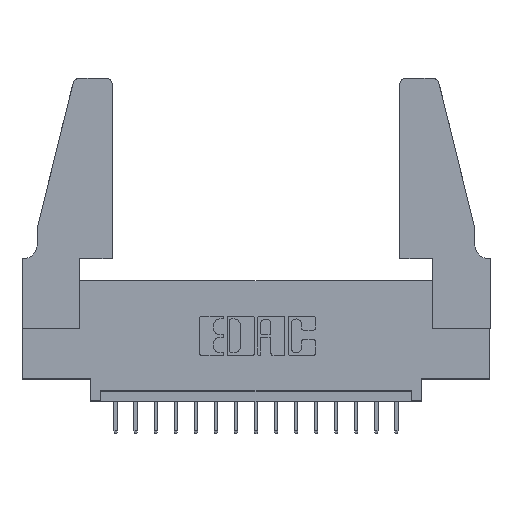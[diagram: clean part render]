
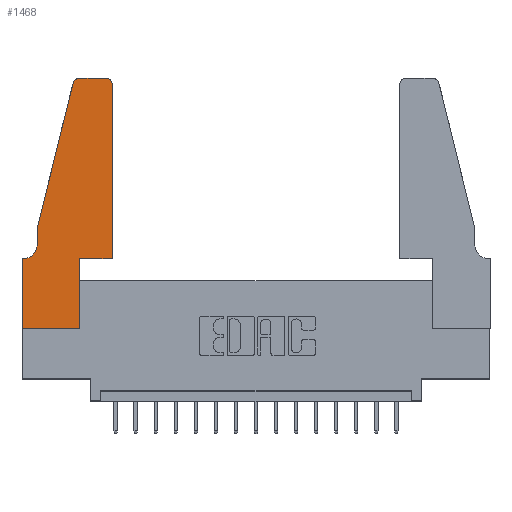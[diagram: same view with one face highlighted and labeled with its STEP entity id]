
A CAD part, top view. The second image highlights one B-rep face of the part: STEP entity #1468.
In plain terms, the highlighted planar face has unit normal (0, 0, 1).
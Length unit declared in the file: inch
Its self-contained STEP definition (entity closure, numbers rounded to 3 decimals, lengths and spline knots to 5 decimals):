
#71 = DIRECTION ( 'NONE',  ( -0.239, -0.971, 0. ) ) ;
#103 = DIRECTION ( 'NONE',  ( 0., 0., 1. ) ) ;
#128 = ORIENTED_EDGE ( 'NONE', *, *, #11020, .T. ) ;
#147 = VERTEX_POINT ( 'NONE', #17184 ) ;
#299 = ORIENTED_EDGE ( 'NONE', *, *, #2047, .T. ) ;
#352 = VERTEX_POINT ( 'NONE', #2187 ) ;
#450 = DIRECTION ( 'NONE',  ( 1., 0., 0. ) ) ;
#629 = EDGE_CURVE ( 'NONE', #147, #1503, #12764, .T. ) ;
#857 = DIRECTION ( 'NONE',  ( 0., 0., 1. ) ) ;
#936 = DIRECTION ( 'NONE',  ( 1., 0., 0. ) ) ;
#990 = VECTOR ( 'NONE', #10093, 39.37008 ) ;
#1235 = DIRECTION ( 'NONE',  ( 0., -1., 0. ) ) ;
#1468 = ADVANCED_FACE ( 'NONE', ( #2275 ), #4804, .T. ) ;
#1503 = VERTEX_POINT ( 'NONE', #3498 ) ;
#1647 = ORIENTED_EDGE ( 'NONE', *, *, #12809, .T. ) ;
#1787 = CARTESIAN_POINT ( 'NONE',  ( 0.0055, 0.42, 0.37 ) ) ;
#2047 = EDGE_CURVE ( 'NONE', #6552, #7746, #2246, .T. ) ;
#2187 = CARTESIAN_POINT ( 'NONE',  ( 0.0755, 0.42, 0.37 ) ) ;
#2246 = LINE ( 'NONE', #8787, #990 ) ;
#2275 = FACE_OUTER_BOUND ( 'NONE', #10332, .T. ) ;
#2312 = CARTESIAN_POINT ( 'NONE',  ( 0.2865, 0.35, 0.37 ) ) ;
#2389 = ORIENTED_EDGE ( 'NONE', *, *, #8992, .T. ) ;
#2421 = EDGE_CURVE ( 'NONE', #13683, #147, #16655, .T. ) ;
#2597 = LINE ( 'NONE', #13970, #16398 ) ;
#2648 = CARTESIAN_POINT ( 'NONE',  ( 0.2865, 0., 0.37 ) ) ;
#3378 = CARTESIAN_POINT ( 'NONE',  ( 0.4505, 0.35, 0.37 ) ) ;
#3498 = CARTESIAN_POINT ( 'NONE',  ( 0.0755, 0.5, 0.37 ) ) ;
#3772 = EDGE_CURVE ( 'NONE', #4771, #9372, #8177, .T. ) ;
#3778 = DIRECTION ( 'NONE',  ( 0., 1., 0. ) ) ;
#4575 = LINE ( 'NONE', #3378, #8749 ) ;
#4703 = VECTOR ( 'NONE', #1235, 39.37008 ) ;
#4771 = VERTEX_POINT ( 'NONE', #2648 ) ;
#4804 = PLANE ( 'NONE',  #5915 ) ;
#5311 = LINE ( 'NONE', #11658, #4703 ) ;
#5514 = VERTEX_POINT ( 'NONE', #15919 ) ;
#5704 = DIRECTION ( 'NONE',  ( -1., 0., 0. ) ) ;
#5915 = AXIS2_PLACEMENT_3D ( 'NONE', #16575, #15476, #12614 ) ;
#6009 = ORIENTED_EDGE ( 'NONE', *, *, #3772, .T. ) ;
#6011 = DIRECTION ( 'NONE',  ( 0., 1., 0. ) ) ;
#6068 = EDGE_CURVE ( 'NONE', #1503, #352, #11899, .T. ) ;
#6233 = CARTESIAN_POINT ( 'NONE',  ( 0.4205, 1.25, 0.37 ) ) ;
#6552 = VERTEX_POINT ( 'NONE', #11330 ) ;
#7275 = VECTOR ( 'NONE', #12005, 39.37008 ) ;
#7746 = VERTEX_POINT ( 'NONE', #14257 ) ;
#7766 = ORIENTED_EDGE ( 'NONE', *, *, #12577, .T. ) ;
#8030 = LINE ( 'NONE', #15045, #17027 ) ;
#8063 = CARTESIAN_POINT ( 'NONE',  ( 0.0755, 0.5, 0.37 ) ) ;
#8177 = LINE ( 'NONE', #2312, #15928 ) ;
#8514 = EDGE_CURVE ( 'NONE', #9424, #4771, #8030, .T. ) ;
#8647 = ORIENTED_EDGE ( 'NONE', *, *, #17154, .T. ) ;
#8749 = VECTOR ( 'NONE', #6011, 39.37008 ) ;
#8785 = CARTESIAN_POINT ( 'NONE',  ( 0., 0., 0.37 ) ) ;
#8787 = CARTESIAN_POINT ( 'NONE',  ( 0.0755, 0.35, 0.37 ) ) ;
#8906 = EDGE_CURVE ( 'NONE', #7746, #9424, #5311, .T. ) ;
#8992 = EDGE_CURVE ( 'NONE', #5514, #9437, #12422, .T. ) ;
#9372 = VERTEX_POINT ( 'NONE', #10990 ) ;
#9424 = VERTEX_POINT ( 'NONE', #8785 ) ;
#9437 = VERTEX_POINT ( 'NONE', #6233 ) ;
#9767 = ORIENTED_EDGE ( 'NONE', *, *, #8906, .T. ) ;
#10093 = DIRECTION ( 'NONE',  ( -1., 0., 0. ) ) ;
#10123 = VERTEX_POINT ( 'NONE', #13968 ) ;
#10332 = EDGE_LOOP ( 'NONE', ( #7766, #13194, #15185, #10929, #128, #299, #9767, #11172, #6009, #1647, #8647, #2389 ) ) ;
#10884 = AXIS2_PLACEMENT_3D ( 'NONE', #14868, #103, #13544 ) ;
#10929 = ORIENTED_EDGE ( 'NONE', *, *, #6068, .T. ) ;
#10990 = CARTESIAN_POINT ( 'NONE',  ( 0.2865, 0.35, 0.37 ) ) ;
#11020 = EDGE_CURVE ( 'NONE', #352, #6552, #15208, .T. ) ;
#11172 = ORIENTED_EDGE ( 'NONE', *, *, #8514, .T. ) ;
#11330 = CARTESIAN_POINT ( 'NONE',  ( 0.0055, 0.35, 0.37 ) ) ;
#11658 = CARTESIAN_POINT ( 'NONE',  ( 0., 0., 0.37 ) ) ;
#11719 = AXIS2_PLACEMENT_3D ( 'NONE', #12835, #857, #14340 ) ;
#11899 = LINE ( 'NONE', #13213, #7275 ) ;
#12005 = DIRECTION ( 'NONE',  ( 0., -1., 0. ) ) ;
#12422 = CIRCLE ( 'NONE', #11719, 0.03 ) ;
#12450 = DIRECTION ( 'NONE',  ( -1., 0., 0. ) ) ;
#12577 = EDGE_CURVE ( 'NONE', #9437, #13683, #14120, .T. ) ;
#12614 = DIRECTION ( 'NONE',  ( 1., 0., 0. ) ) ;
#12764 = LINE ( 'NONE', #8063, #13160 ) ;
#12809 = EDGE_CURVE ( 'NONE', #9372, #10123, #2597, .T. ) ;
#12835 = CARTESIAN_POINT ( 'NONE',  ( 0.4205, 1.22, 0.37 ) ) ;
#13160 = VECTOR ( 'NONE', #71, 39.37008 ) ;
#13194 = ORIENTED_EDGE ( 'NONE', *, *, #2421, .T. ) ;
#13213 = CARTESIAN_POINT ( 'NONE',  ( 0.0755, 0.5, 0.37 ) ) ;
#13544 = DIRECTION ( 'NONE',  ( 1., 0., 0. ) ) ;
#13616 = CARTESIAN_POINT ( 'NONE',  ( 0.2605, 1.25, 0.37 ) ) ;
#13683 = VERTEX_POINT ( 'NONE', #17244 ) ;
#13968 = CARTESIAN_POINT ( 'NONE',  ( 0.4505, 0.35, 0.37 ) ) ;
#13970 = CARTESIAN_POINT ( 'NONE',  ( 0.4505, 0.35, 0.37 ) ) ;
#14120 = LINE ( 'NONE', #13616, #16625 ) ;
#14257 = CARTESIAN_POINT ( 'NONE',  ( 0., 0.35, 0.37 ) ) ;
#14340 = DIRECTION ( 'NONE',  ( 1., 0., 0. ) ) ;
#14868 = CARTESIAN_POINT ( 'NONE',  ( 0.284, 1.22, 0.37 ) ) ;
#15045 = CARTESIAN_POINT ( 'NONE',  ( 0., 0., 0.37 ) ) ;
#15163 = DIRECTION ( 'NONE',  ( 0., 0., -1. ) ) ;
#15185 = ORIENTED_EDGE ( 'NONE', *, *, #629, .T. ) ;
#15208 = CIRCLE ( 'NONE', #16759, 0.07 ) ;
#15476 = DIRECTION ( 'NONE',  ( 0., 0., 1. ) ) ;
#15919 = CARTESIAN_POINT ( 'NONE',  ( 0.4505, 1.22, 0.37 ) ) ;
#15928 = VECTOR ( 'NONE', #3778, 39.37008 ) ;
#16398 = VECTOR ( 'NONE', #936, 39.37008 ) ;
#16575 = CARTESIAN_POINT ( 'NONE',  ( 0., 0.35, 0.37 ) ) ;
#16625 = VECTOR ( 'NONE', #12450, 39.37008 ) ;
#16655 = CIRCLE ( 'NONE', #10884, 0.03 ) ;
#16759 = AXIS2_PLACEMENT_3D ( 'NONE', #1787, #15163, #5704 ) ;
#17027 = VECTOR ( 'NONE', #450, 39.37008 ) ;
#17154 = EDGE_CURVE ( 'NONE', #10123, #5514, #4575, .T. ) ;
#17184 = CARTESIAN_POINT ( 'NONE',  ( 0.25487, 1.22718, 0.37 ) ) ;
#17244 = CARTESIAN_POINT ( 'NONE',  ( 0.284, 1.25, 0.37 ) ) ;
